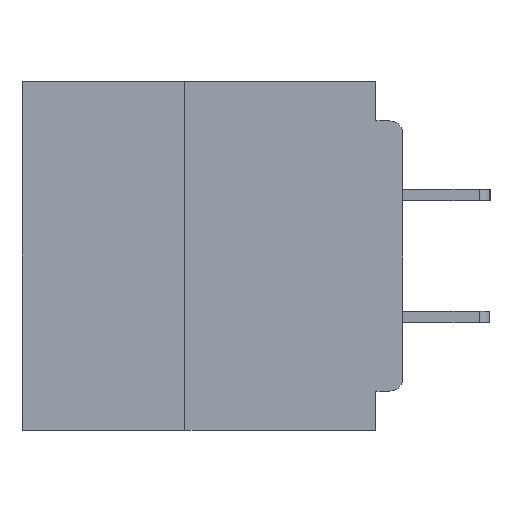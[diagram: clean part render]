
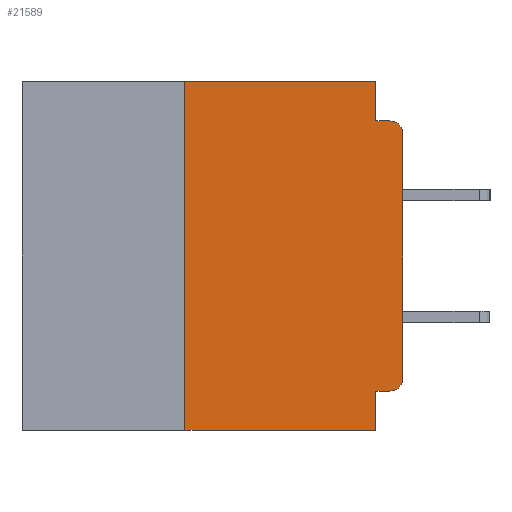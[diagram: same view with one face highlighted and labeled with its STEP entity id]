
A CAD part, left-side view. The second image highlights one B-rep face of the part: STEP entity #21589.
In plain terms, the highlighted planar face has unit normal (-1, 0, 0).
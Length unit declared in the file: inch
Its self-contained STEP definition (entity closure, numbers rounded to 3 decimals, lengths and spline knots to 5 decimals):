
#541 = CARTESIAN_POINT ( 'NONE',  ( 0., 0.25, -0.4 ) ) ;
#733 = LINE ( 'NONE', #12168, #36893 ) ;
#840 = AXIS2_PLACEMENT_3D ( 'NONE', #28303, #28262, #28228 ) ;
#1121 = VERTEX_POINT ( 'NONE', #18400 ) ;
#1552 = LINE ( 'NONE', #16179, #14496 ) ;
#1736 = LINE ( 'NONE', #34403, #16494 ) ;
#2698 = DIRECTION ( 'NONE',  ( 0., 0., -1. ) ) ;
#2821 = DIRECTION ( 'NONE',  ( -1., 0., 0. ) ) ;
#2897 = CARTESIAN_POINT ( 'NONE',  ( 0., 0.015, -0.06 ) ) ;
#2942 = CARTESIAN_POINT ( 'NONE',  ( 0., 0.031, -0.4 ) ) ;
#4201 = EDGE_CURVE ( 'NONE', #16819, #22871, #28129, .T. ) ;
#5159 = LINE ( 'NONE', #25504, #35390 ) ;
#5572 = LINE ( 'NONE', #6402, #21211 ) ;
#6402 = CARTESIAN_POINT ( 'NONE',  ( 0., 0., 0. ) ) ;
#6472 = DIRECTION ( 'NONE',  ( 0., 1., 0. ) ) ;
#6554 = EDGE_CURVE ( 'NONE', #8770, #18409, #9909, .T. ) ;
#7290 = VECTOR ( 'NONE', #6472, 39.37008 ) ;
#7360 = DIRECTION ( 'NONE',  ( 0., -1., 0. ) ) ;
#8770 = VERTEX_POINT ( 'NONE', #10095 ) ;
#9772 = DIRECTION ( 'NONE',  ( 1., 0., 0. ) ) ;
#9909 = CIRCLE ( 'NONE', #17245, 0.015 ) ;
#10095 = CARTESIAN_POINT ( 'NONE',  ( 0., 0., -0.06 ) ) ;
#10134 = LINE ( 'NONE', #2942, #17035 ) ;
#10915 = CARTESIAN_POINT ( 'NONE',  ( 0., 0.015, -0.045 ) ) ;
#11093 = ORIENTED_EDGE ( 'NONE', *, *, #4201, .T. ) ;
#11260 = ORIENTED_EDGE ( 'NONE', *, *, #23767, .F. ) ;
#12168 = CARTESIAN_POINT ( 'NONE',  ( 0., 0.437, -0.4 ) ) ;
#12302 = ORIENTED_EDGE ( 'NONE', *, *, #34268, .F. ) ;
#13209 = VERTEX_POINT ( 'NONE', #28611 ) ;
#14353 = ORIENTED_EDGE ( 'NONE', *, *, #19309, .T. ) ;
#14496 = VECTOR ( 'NONE', #7360, 39.37008 ) ;
#15216 = LINE ( 'NONE', #24027, #7290 ) ;
#16179 = CARTESIAN_POINT ( 'NONE',  ( 0., 0.437, 0. ) ) ;
#16494 = VECTOR ( 'NONE', #37271, 39.37008 ) ;
#16819 = VERTEX_POINT ( 'NONE', #35269 ) ;
#16887 = VERTEX_POINT ( 'NONE', #32704 ) ;
#17035 = VECTOR ( 'NONE', #17615, 39.37008 ) ;
#17245 = AXIS2_PLACEMENT_3D ( 'NONE', #2897, #2821, #2698 ) ;
#17587 = ORIENTED_EDGE ( 'NONE', *, *, #6554, .T. ) ;
#17615 = DIRECTION ( 'NONE',  ( 0., 0., -1. ) ) ;
#18400 = CARTESIAN_POINT ( 'NONE',  ( 0., 0.031, -0.355 ) ) ;
#18409 = VERTEX_POINT ( 'NONE', #10915 ) ;
#18768 = AXIS2_PLACEMENT_3D ( 'NONE', #27297, #9772, #30229 ) ;
#19309 = EDGE_CURVE ( 'NONE', #36371, #33442, #733, .T. ) ;
#20235 = EDGE_LOOP ( 'NONE', ( #21746, #17587, #21951, #12302, #33809, #25886, #14353, #11260, #28732, #11093 ) ) ;
#21211 = VECTOR ( 'NONE', #32777, 39.37008 ) ;
#21444 = PLANE ( 'NONE',  #18768 ) ;
#21589 = ADVANCED_FACE ( 'NONE', ( #26760 ), #21444, .F. ) ;
#21746 = ORIENTED_EDGE ( 'NONE', *, *, #30737, .T. ) ;
#21951 = ORIENTED_EDGE ( 'NONE', *, *, #24817, .F. ) ;
#21978 = VECTOR ( 'NONE', #29913, 39.37008 ) ;
#22871 = VERTEX_POINT ( 'NONE', #36722 ) ;
#23767 = EDGE_CURVE ( 'NONE', #1121, #33442, #10134, .T. ) ;
#24027 = CARTESIAN_POINT ( 'NONE',  ( 0., 0., -0.355 ) ) ;
#24817 = EDGE_CURVE ( 'NONE', #13209, #18409, #1736, .T. ) ;
#25504 = CARTESIAN_POINT ( 'NONE',  ( 0., 0.031, 0. ) ) ;
#25886 = ORIENTED_EDGE ( 'NONE', *, *, #34867, .F. ) ;
#26138 = CARTESIAN_POINT ( 'NONE',  ( 0., 0.25, 0. ) ) ;
#26760 = FACE_OUTER_BOUND ( 'NONE', #20235, .T. ) ;
#27297 = CARTESIAN_POINT ( 'NONE',  ( 0., 0.437, 0. ) ) ;
#28129 = CIRCLE ( 'NONE', #840, 0.015 ) ;
#28228 = DIRECTION ( 'NONE',  ( 0., 0., -1. ) ) ;
#28262 = DIRECTION ( 'NONE',  ( -1., 0., 0. ) ) ;
#28303 = CARTESIAN_POINT ( 'NONE',  ( 0., 0.015, -0.34 ) ) ;
#28479 = VERTEX_POINT ( 'NONE', #26138 ) ;
#28611 = CARTESIAN_POINT ( 'NONE',  ( 0., 0.031, -0.045 ) ) ;
#28732 = ORIENTED_EDGE ( 'NONE', *, *, #34861, .F. ) ;
#29454 = CARTESIAN_POINT ( 'NONE',  ( 0., 0.25, -0.4 ) ) ;
#29647 = DIRECTION ( 'NONE',  ( 0., -1., 0. ) ) ;
#29755 = LINE ( 'NONE', #541, #21978 ) ;
#29913 = DIRECTION ( 'NONE',  ( 0., 0., 1. ) ) ;
#30229 = DIRECTION ( 'NONE',  ( 0., 0., -1. ) ) ;
#30737 = EDGE_CURVE ( 'NONE', #22871, #8770, #5572, .T. ) ;
#31504 = DIRECTION ( 'NONE',  ( 0., 0., -1. ) ) ;
#31911 = CARTESIAN_POINT ( 'NONE',  ( 0., 0.031, -0.4 ) ) ;
#32704 = CARTESIAN_POINT ( 'NONE',  ( 0., 0.031, 0. ) ) ;
#32777 = DIRECTION ( 'NONE',  ( 0., 0., 1. ) ) ;
#33442 = VERTEX_POINT ( 'NONE', #31911 ) ;
#33809 = ORIENTED_EDGE ( 'NONE', *, *, #37252, .F. ) ;
#34268 = EDGE_CURVE ( 'NONE', #16887, #13209, #5159, .T. ) ;
#34403 = CARTESIAN_POINT ( 'NONE',  ( 0., 0., -0.045 ) ) ;
#34861 = EDGE_CURVE ( 'NONE', #16819, #1121, #15216, .T. ) ;
#34867 = EDGE_CURVE ( 'NONE', #36371, #28479, #29755, .T. ) ;
#35269 = CARTESIAN_POINT ( 'NONE',  ( 0., 0.015, -0.355 ) ) ;
#35390 = VECTOR ( 'NONE', #31504, 39.37008 ) ;
#36371 = VERTEX_POINT ( 'NONE', #29454 ) ;
#36722 = CARTESIAN_POINT ( 'NONE',  ( 0., 0., -0.34 ) ) ;
#36893 = VECTOR ( 'NONE', #29647, 39.37008 ) ;
#37252 = EDGE_CURVE ( 'NONE', #28479, #16887, #1552, .T. ) ;
#37271 = DIRECTION ( 'NONE',  ( 0., -1., 0. ) ) ;
